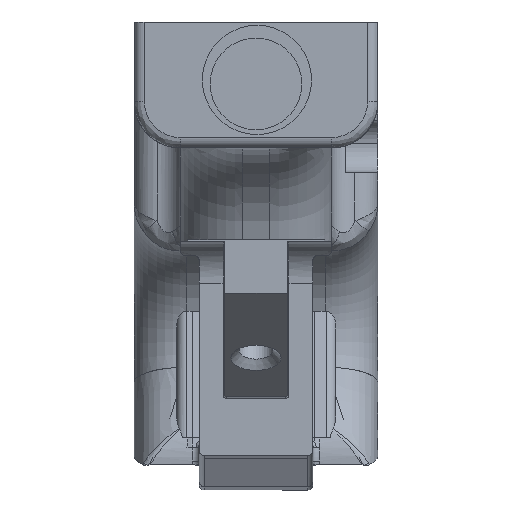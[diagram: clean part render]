
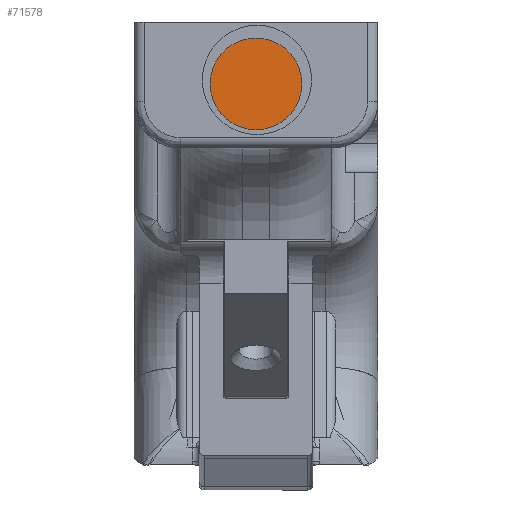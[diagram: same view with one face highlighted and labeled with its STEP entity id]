
A CAD part, left-side view. The second image highlights one B-rep face of the part: STEP entity #71578.
In plain terms, the highlighted planar face has unit normal (-1, 0, 0).
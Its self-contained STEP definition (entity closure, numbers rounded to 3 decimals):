
#31386 = PLANE('',#31387);
#31387 = AXIS2_PLACEMENT_3D('',#31388,#31389,#31390);
#31388 = CARTESIAN_POINT('',(-27.367,102.106,154.638)
  );
#31389 = DIRECTION('',(1.,0.,0.));
#31390 = DIRECTION('',(0.,0.,1.));
#55440 = EDGE_CURVE('',#55441,#55441,#55443,.T.);
#55441 = VERTEX_POINT('',#55442);
#55442 = CARTESIAN_POINT('',(-27.367,110.574,
    147.046));
#55443 = SURFACE_CURVE('',#55444,(#55449,#55456),.PCURVE_S1.);
#55444 = CIRCLE('',#55445,6.985);
#55445 = AXIS2_PLACEMENT_3D('',#55446,#55447,#55448);
#55446 = CARTESIAN_POINT('',(-27.367,110.574,
    154.031));
#55447 = DIRECTION('',(1.,0.,0.));
#55448 = DIRECTION('',(0.,0.,-1.));
#55449 = PCURVE('',#31386,#55450);
#55450 = DEFINITIONAL_REPRESENTATION('',(#55451),#55455);
#55451 = CIRCLE('',#55452,6.985);
#55452 = AXIS2_PLACEMENT_2D('',#55453,#55454);
#55453 = CARTESIAN_POINT('',(-0.608,-8.468));
#55454 = DIRECTION('',(-1.,0.));
#55455 = ( GEOMETRIC_REPRESENTATION_CONTEXT(2) 
PARAMETRIC_REPRESENTATION_CONTEXT() REPRESENTATION_CONTEXT('2D SPACE',''
  ) );
#55456 = PCURVE('',#55457,#55462);
#55457 = PLANE('',#55458);
#55458 = AXIS2_PLACEMENT_3D('',#55459,#55460,#55461);
#55459 = CARTESIAN_POINT('',(-27.367,102.106,154.638)
  );
#55460 = DIRECTION('',(1.,0.,0.));
#55461 = DIRECTION('',(0.,0.,1.));
#55462 = DEFINITIONAL_REPRESENTATION('',(#55463),#55467);
#55463 = CIRCLE('',#55464,6.985);
#55464 = AXIS2_PLACEMENT_2D('',#55465,#55466);
#55465 = CARTESIAN_POINT('',(-0.608,-8.468));
#55466 = DIRECTION('',(-1.,0.));
#55467 = ( GEOMETRIC_REPRESENTATION_CONTEXT(2) 
PARAMETRIC_REPRESENTATION_CONTEXT() REPRESENTATION_CONTEXT('2D SPACE',''
  ) );
#71578 = ADVANCED_FACE('',(#71579),#55457,.F.);
#71579 = FACE_BOUND('',#71580,.F.);
#71580 = EDGE_LOOP('',(#71581));
#71581 = ORIENTED_EDGE('',*,*,#55440,.T.);
